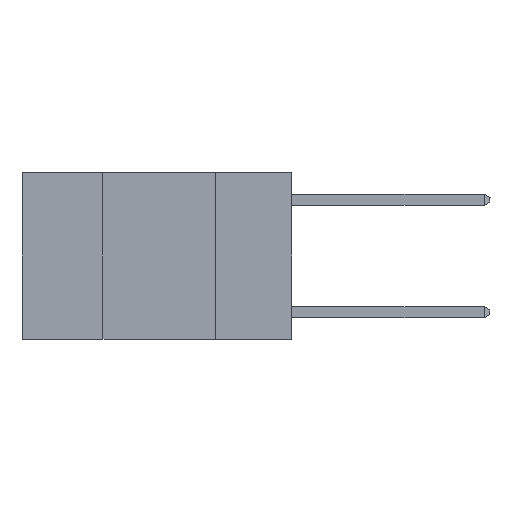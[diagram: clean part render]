
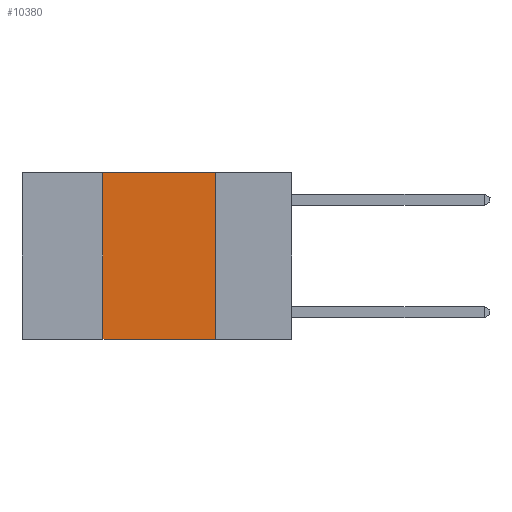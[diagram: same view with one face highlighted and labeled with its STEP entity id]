
A CAD part, left-side view. The second image highlights one B-rep face of the part: STEP entity #10380.
In plain terms, the highlighted planar face has unit normal (-1, 0, 0).
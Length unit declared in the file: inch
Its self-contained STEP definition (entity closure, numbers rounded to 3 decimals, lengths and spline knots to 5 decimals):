
#619 = DIRECTION ( 'NONE',  ( 0., -1., 0. ) ) ;
#965 = EDGE_CURVE ( 'NONE', #6027, #2131, #6698, .T. ) ;
#1117 = CARTESIAN_POINT ( 'NONE',  ( 0., 0.42, 0. ) ) ;
#1402 = DIRECTION ( 'NONE',  ( 0., 0., -1. ) ) ;
#1475 = FACE_OUTER_BOUND ( 'NONE', #7111, .T. ) ;
#2125 = CARTESIAN_POINT ( 'NONE',  ( 0., 0.42, -0.37 ) ) ;
#2131 = VERTEX_POINT ( 'NONE', #6266 ) ;
#2278 = DIRECTION ( 'NONE',  ( 0., 0., -1. ) ) ;
#2286 = VERTEX_POINT ( 'NONE', #2125 ) ;
#2525 = VECTOR ( 'NONE', #8089, 39.37008 ) ;
#2597 = VECTOR ( 'NONE', #9896, 39.37008 ) ;
#2734 = EDGE_CURVE ( 'NONE', #2131, #5175, #9177, .T. ) ;
#2846 = EDGE_CURVE ( 'NONE', #2286, #6027, #4545, .T. ) ;
#2867 = VECTOR ( 'NONE', #1402, 39.37008 ) ;
#3108 = PLANE ( 'NONE',  #4018 ) ;
#3182 = CARTESIAN_POINT ( 'NONE',  ( 0., 0.6, -0.37 ) ) ;
#3582 = CARTESIAN_POINT ( 'NONE',  ( 0., 0.42, 0. ) ) ;
#4018 = AXIS2_PLACEMENT_3D ( 'NONE', #9993, #6695, #2278 ) ;
#4545 = LINE ( 'NONE', #1117, #2525 ) ;
#5175 = VERTEX_POINT ( 'NONE', #10443 ) ;
#5472 = ORIENTED_EDGE ( 'NONE', *, *, #9897, .T. ) ;
#5738 = CARTESIAN_POINT ( 'NONE',  ( 0., 0.6, 0. ) ) ;
#6027 = VERTEX_POINT ( 'NONE', #3582 ) ;
#6266 = CARTESIAN_POINT ( 'NONE',  ( 0., 0.17, 0. ) ) ;
#6695 = DIRECTION ( 'NONE',  ( 1., 0., 0. ) ) ;
#6698 = LINE ( 'NONE', #5738, #6807 ) ;
#6807 = VECTOR ( 'NONE', #619, 39.37008 ) ;
#7111 = EDGE_LOOP ( 'NONE', ( #8993, #7475, #9185, #5472 ) ) ;
#7475 = ORIENTED_EDGE ( 'NONE', *, *, #965, .F. ) ;
#7483 = CARTESIAN_POINT ( 'NONE',  ( 0., 0.17, 0. ) ) ;
#8089 = DIRECTION ( 'NONE',  ( 0., 0., 1. ) ) ;
#8993 = ORIENTED_EDGE ( 'NONE', *, *, #2734, .F. ) ;
#9052 = LINE ( 'NONE', #3182, #2597 ) ;
#9177 = LINE ( 'NONE', #7483, #2867 ) ;
#9185 = ORIENTED_EDGE ( 'NONE', *, *, #2846, .F. ) ;
#9897 = EDGE_CURVE ( 'NONE', #2286, #5175, #9052, .T. ) ;
#9896 = DIRECTION ( 'NONE',  ( 0., -1., 0. ) ) ;
#9993 = CARTESIAN_POINT ( 'NONE',  ( 0., 0.6, 0. ) ) ;
#10380 = ADVANCED_FACE ( 'NONE', ( #1475 ), #3108, .F. ) ;
#10443 = CARTESIAN_POINT ( 'NONE',  ( 0., 0.17, -0.37 ) ) ;
